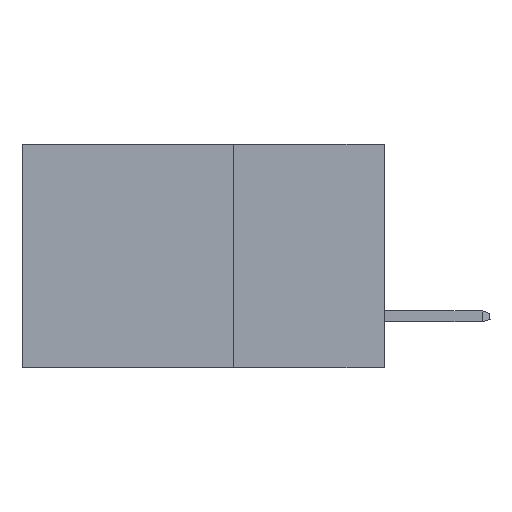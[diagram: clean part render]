
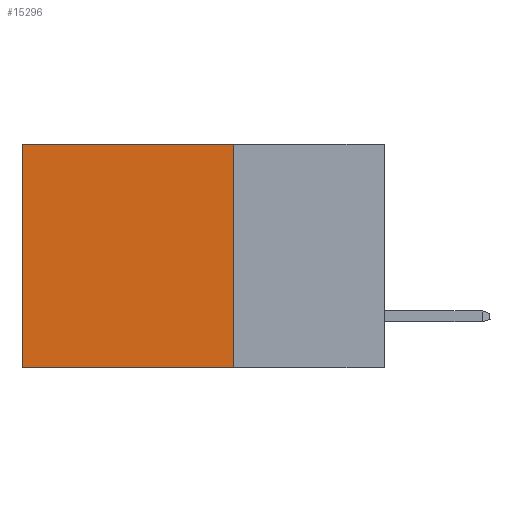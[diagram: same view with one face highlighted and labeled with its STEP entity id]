
A CAD part, left-side view. The second image highlights one B-rep face of the part: STEP entity #15296.
In plain terms, the highlighted planar face has unit normal (-1, 0, 0).
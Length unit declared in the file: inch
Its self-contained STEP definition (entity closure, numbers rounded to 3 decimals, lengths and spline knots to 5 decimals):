
#1584 = AXIS2_PLACEMENT_3D ( 'NONE', #2851, #10093, #26513 ) ;
#2851 = CARTESIAN_POINT ( 'NONE',  ( 0.298, 0.25, 0. ) ) ;
#3016 = EDGE_CURVE ( 'NONE', #12723, #30160, #18088, .T. ) ;
#5436 = VECTOR ( 'NONE', #6456, 39.37008 ) ;
#6104 = ORIENTED_EDGE ( 'NONE', *, *, #13554, .T. ) ;
#6456 = DIRECTION ( 'NONE',  ( 0., 0., -1. ) ) ;
#7587 = ORIENTED_EDGE ( 'NONE', *, *, #3016, .F. ) ;
#7835 = CARTESIAN_POINT ( 'NONE',  ( 0.298, 0.25, 0. ) ) ;
#8065 = VECTOR ( 'NONE', #22558, 39.37008 ) ;
#8519 = CARTESIAN_POINT ( 'NONE',  ( 0.298, 0.25, -0.37 ) ) ;
#8558 = CARTESIAN_POINT ( 'NONE',  ( 0.298, 0.6, -0.37 ) ) ;
#9479 = VECTOR ( 'NONE', #10927, 39.37008 ) ;
#9924 = FACE_OUTER_BOUND ( 'NONE', #22834, .T. ) ;
#10093 = DIRECTION ( 'NONE',  ( 1., 0., 0. ) ) ;
#10927 = DIRECTION ( 'NONE',  ( 0., 1., 0. ) ) ;
#11100 = ORIENTED_EDGE ( 'NONE', *, *, #20734, .T. ) ;
#11579 = VERTEX_POINT ( 'NONE', #8558 ) ;
#12282 = EDGE_CURVE ( 'NONE', #30160, #11579, #22009, .T. ) ;
#12723 = VERTEX_POINT ( 'NONE', #7835 ) ;
#13389 = DIRECTION ( 'NONE',  ( 0., 0., -1. ) ) ;
#13554 = EDGE_CURVE ( 'NONE', #16967, #11579, #14191, .T. ) ;
#14191 = LINE ( 'NONE', #29800, #19728 ) ;
#15296 = ADVANCED_FACE ( 'NONE', ( #9924 ), #24192, .F. ) ;
#16967 = VERTEX_POINT ( 'NONE', #27600 ) ;
#18088 = LINE ( 'NONE', #23020, #5436 ) ;
#19728 = VECTOR ( 'NONE', #13389, 39.37008 ) ;
#20100 = ORIENTED_EDGE ( 'NONE', *, *, #12282, .F. ) ;
#20181 = CARTESIAN_POINT ( 'NONE',  ( 0.298, 0.25, 0. ) ) ;
#20734 = EDGE_CURVE ( 'NONE', #12723, #16967, #27602, .T. ) ;
#22009 = LINE ( 'NONE', #8519, #9479 ) ;
#22558 = DIRECTION ( 'NONE',  ( 0., 1., 0. ) ) ;
#22834 = EDGE_LOOP ( 'NONE', ( #6104, #20100, #7587, #11100 ) ) ;
#23020 = CARTESIAN_POINT ( 'NONE',  ( 0.298, 0.25, 0. ) ) ;
#24192 = PLANE ( 'NONE',  #1584 ) ;
#25945 = CARTESIAN_POINT ( 'NONE',  ( 0.298, 0.25, -0.37 ) ) ;
#26513 = DIRECTION ( 'NONE',  ( 0., 0., -1. ) ) ;
#27600 = CARTESIAN_POINT ( 'NONE',  ( 0.298, 0.6, 0. ) ) ;
#27602 = LINE ( 'NONE', #20181, #8065 ) ;
#29800 = CARTESIAN_POINT ( 'NONE',  ( 0.298, 0.6, 0. ) ) ;
#30160 = VERTEX_POINT ( 'NONE', #25945 ) ;
